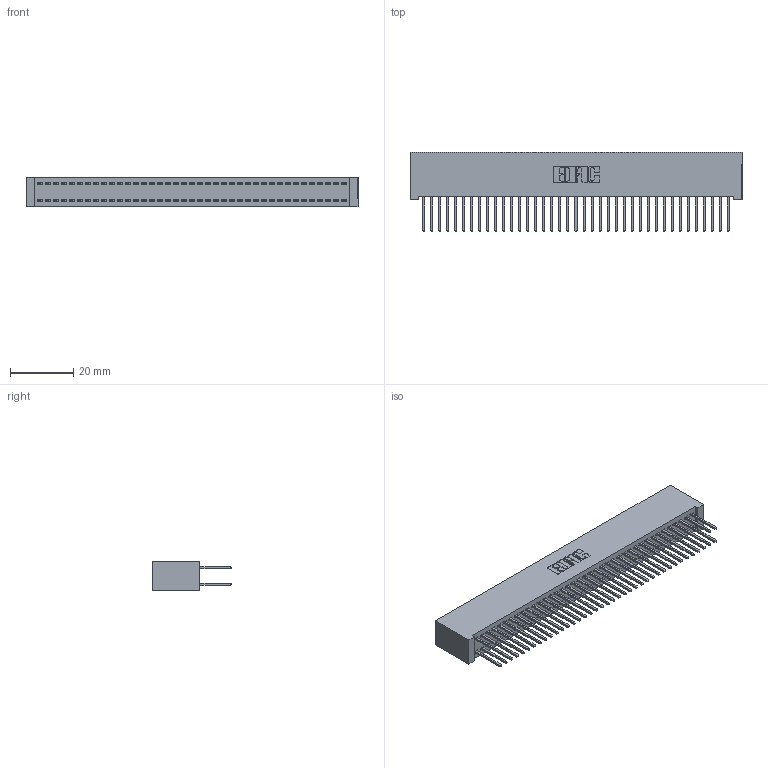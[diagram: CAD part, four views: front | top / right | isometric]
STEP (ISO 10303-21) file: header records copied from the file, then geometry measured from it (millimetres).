
FILE_DESCRIPTION (( 'STEP AP203' ), '1' );
FILE_NAME ('392-078-523-201.STEP', '2019-10-09T13:53:23', ( '' ), ( '' ), 'SwSTEP 2.0', 'SolidWorks 2016', '' );
FILE_SCHEMA (( 'CONFIG_CONTROL_DESIGN' ));
Length unit declared in the file: inch
Products named in the file (3): 342 Part_Lugless; 345-292-001_345-293-123; 392-078-523-201
Assembly tree (79 placements, depth 2):
  392-078-523-201
    342 Part_Lugless
    345-292-001_345-293-123  x78
Bounding box: 105.31 x 25.15 x 9.4 mm (x, y, z)
Volume: 10047.1 mm3; surface area: 17406.7 mm2
Topology: 79 solids, 79 shells, 4158 faces, 12365 edges, 8138 vertices
Faces by surface type: plane 2870, cylinder 1288
Entity records: 25087 total; most frequent: CARTESIAN_POINT 4158, ORIENTED_EDGE 4094, DIRECTION 3551, EDGE_CURVE 2047, VECTOR 1927, LINE 1927, VERTEX_POINT 1362, AXIS2_PLACEMENT_3D 812
